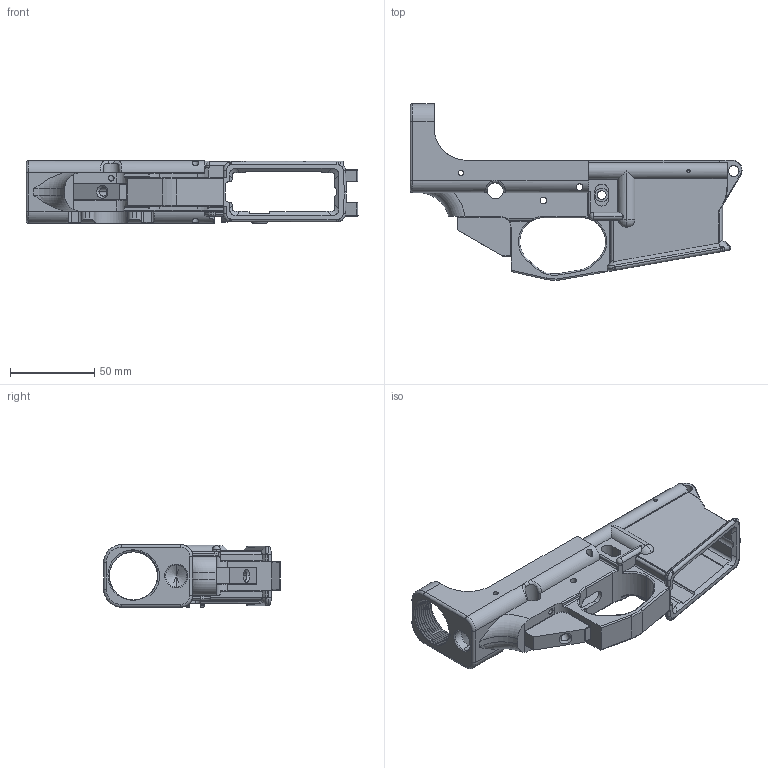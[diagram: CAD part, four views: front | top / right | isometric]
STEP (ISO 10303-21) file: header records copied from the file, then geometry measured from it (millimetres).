
FILE_DESCRIPTION (( 'STEP AP214' ), '1' );
FILE_NAME ('AR-15 - Lower Receiver DD - WW REV 3.3.1-Test 1 (jad).STEP', '' );
FILE_SCHEMA (( 'AUTOMOTIVE_DESIGN' ));
Length unit declared in the file: inch
Products named in the file (1): AR-15 - Lower Receiver DD - WW REV 3.3.1-Test 1 (jad)
Bounding box: 197.08 x 104.92 x 37.19 mm (x, y, z)
Volume: 134375.2 mm3; surface area: 58188.9 mm2
Topology: 1 solids, 1 shells, 871 faces, 2377 edges, 1525 vertices
Faces by surface type: plane 394, cylinder 251, bspline 154, torus 53, cone 12, sphere 7
Entity records: 54818 total; most frequent: CARTESIAN_POINT 34179, ORIENTED_EDGE 4730, DIRECTION 3656, EDGE_CURVE 2365, VERTEX_POINT 1525, LINE 1374, VECTOR 1374, AXIS2_PLACEMENT_3D 1141
